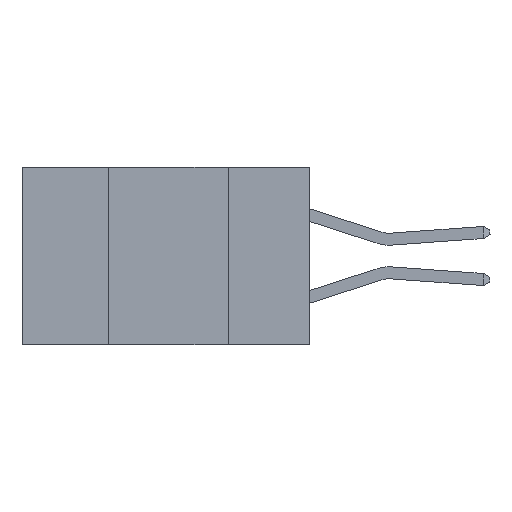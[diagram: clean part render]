
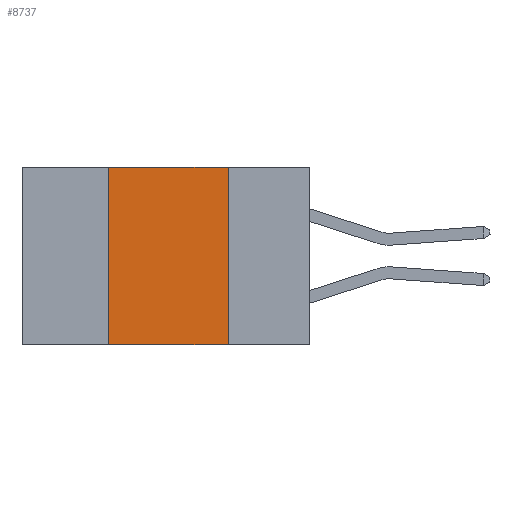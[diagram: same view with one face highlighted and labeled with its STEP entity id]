
A CAD part, left-side view. The second image highlights one B-rep face of the part: STEP entity #8737.
In plain terms, the highlighted planar face has unit normal (-1, 0, 0).
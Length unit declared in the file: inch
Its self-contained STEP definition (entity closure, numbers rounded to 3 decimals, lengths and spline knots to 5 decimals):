
#288 = PLANE ( 'NONE',  #5032 ) ;
#491 = ORIENTED_EDGE ( 'NONE', *, *, #3273, .F. ) ;
#1465 = LINE ( 'NONE', #12397, #3547 ) ;
#2121 = EDGE_CURVE ( 'NONE', #3236, #9478, #7393, .T. ) ;
#2362 = VECTOR ( 'NONE', #7323, 39.37008 ) ;
#2796 = CARTESIAN_POINT ( 'NONE',  ( 0., 0.6, -0.37 ) ) ;
#3188 = ORIENTED_EDGE ( 'NONE', *, *, #11586, .F. ) ;
#3236 = VERTEX_POINT ( 'NONE', #10890 ) ;
#3273 = EDGE_CURVE ( 'NONE', #6758, #9478, #1465, .T. ) ;
#3547 = VECTOR ( 'NONE', #5824, 39.37008 ) ;
#3609 = FACE_OUTER_BOUND ( 'NONE', #12638, .T. ) ;
#4612 = DIRECTION ( 'NONE',  ( 1., 0., 0. ) ) ;
#4971 = CARTESIAN_POINT ( 'NONE',  ( 0., 0.42, -0.37 ) ) ;
#5020 = VECTOR ( 'NONE', #9331, 39.37008 ) ;
#5032 = AXIS2_PLACEMENT_3D ( 'NONE', #13531, #4612, #5892 ) ;
#5824 = DIRECTION ( 'NONE',  ( 0., 0., -1. ) ) ;
#5892 = DIRECTION ( 'NONE',  ( 0., 0., -1. ) ) ;
#6758 = VERTEX_POINT ( 'NONE', #8991 ) ;
#7323 = DIRECTION ( 'NONE',  ( 0., -1., 0. ) ) ;
#7393 = LINE ( 'NONE', #2796, #2362 ) ;
#7936 = ORIENTED_EDGE ( 'NONE', *, *, #8256, .F. ) ;
#8019 = ORIENTED_EDGE ( 'NONE', *, *, #2121, .T. ) ;
#8256 = EDGE_CURVE ( 'NONE', #3236, #10059, #12670, .T. ) ;
#8737 = ADVANCED_FACE ( 'NONE', ( #3609 ), #288, .F. ) ;
#8991 = CARTESIAN_POINT ( 'NONE',  ( 0., 0.17, 0. ) ) ;
#9331 = DIRECTION ( 'NONE',  ( 0., 0., 1. ) ) ;
#9398 = DIRECTION ( 'NONE',  ( 0., -1., 0. ) ) ;
#9478 = VERTEX_POINT ( 'NONE', #13236 ) ;
#9609 = CARTESIAN_POINT ( 'NONE',  ( 0., 0.6, 0. ) ) ;
#10059 = VERTEX_POINT ( 'NONE', #12098 ) ;
#10393 = LINE ( 'NONE', #9609, #11935 ) ;
#10890 = CARTESIAN_POINT ( 'NONE',  ( 0., 0.42, -0.37 ) ) ;
#11586 = EDGE_CURVE ( 'NONE', #10059, #6758, #10393, .T. ) ;
#11935 = VECTOR ( 'NONE', #9398, 39.37008 ) ;
#12098 = CARTESIAN_POINT ( 'NONE',  ( 0., 0.42, 0. ) ) ;
#12397 = CARTESIAN_POINT ( 'NONE',  ( 0., 0.17, -0.37 ) ) ;
#12638 = EDGE_LOOP ( 'NONE', ( #491, #3188, #7936, #8019 ) ) ;
#12670 = LINE ( 'NONE', #4971, #5020 ) ;
#13236 = CARTESIAN_POINT ( 'NONE',  ( 0., 0.17, -0.37 ) ) ;
#13531 = CARTESIAN_POINT ( 'NONE',  ( 0., 0.6, 0. ) ) ;
